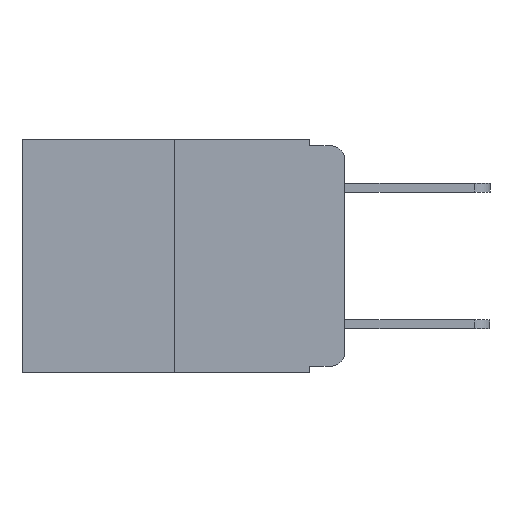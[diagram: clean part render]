
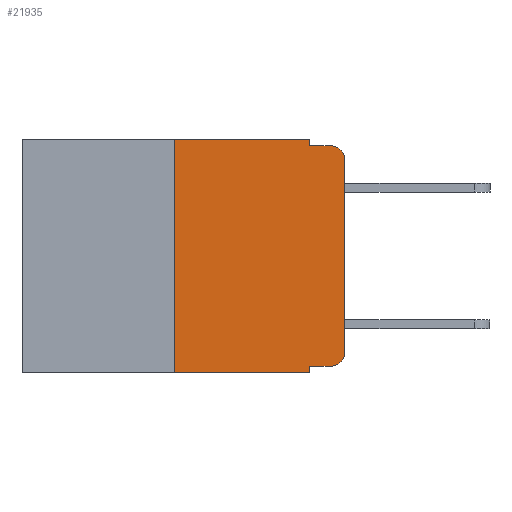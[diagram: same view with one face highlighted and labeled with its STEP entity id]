
A CAD part, left-side view. The second image highlights one B-rep face of the part: STEP entity #21935.
In plain terms, the highlighted planar face has unit normal (-1, 0, 0).
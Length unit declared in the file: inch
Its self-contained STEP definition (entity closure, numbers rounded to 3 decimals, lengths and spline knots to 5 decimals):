
#330 = ORIENTED_EDGE ( 'NONE', *, *, #23848, .F. ) ;
#462 = ORIENTED_EDGE ( 'NONE', *, *, #19338, .F. ) ;
#585 = CARTESIAN_POINT ( 'NONE',  ( 0., 0.051, -0.333 ) ) ;
#984 = ORIENTED_EDGE ( 'NONE', *, *, #8933, .F. ) ;
#1014 = AXIS2_PLACEMENT_3D ( 'NONE', #10440, #23750, #12468 ) ;
#1226 = ORIENTED_EDGE ( 'NONE', *, *, #25262, .T. ) ;
#1293 = ORIENTED_EDGE ( 'NONE', *, *, #23496, .F. ) ;
#1392 = VERTEX_POINT ( 'NONE', #13499 ) ;
#1711 = CARTESIAN_POINT ( 'NONE',  ( 0., 0.25, 0. ) ) ;
#1817 = ORIENTED_EDGE ( 'NONE', *, *, #15068, .F. ) ;
#2026 = DIRECTION ( 'NONE',  ( 0., -1., 0. ) ) ;
#2485 = EDGE_CURVE ( 'NONE', #4805, #18798, #21576, .T. ) ;
#2813 = CARTESIAN_POINT ( 'NONE',  ( 0., 0.051, -0.333 ) ) ;
#2828 = VERTEX_POINT ( 'NONE', #23928 ) ;
#3461 = DIRECTION ( 'NONE',  ( 0., 0., 1. ) ) ;
#3633 = ORIENTED_EDGE ( 'NONE', *, *, #18887, .T. ) ;
#3906 = CARTESIAN_POINT ( 'NONE',  ( 0., 0.051, -0.343 ) ) ;
#4302 = CARTESIAN_POINT ( 'NONE',  ( 0., 0.051, -0.01 ) ) ;
#4327 = LINE ( 'NONE', #13667, #20032 ) ;
#4404 = DIRECTION ( 'NONE',  ( 0., -1., 0. ) ) ;
#4767 = CARTESIAN_POINT ( 'NONE',  ( 0., 0.02, -0.333 ) ) ;
#4805 = VERTEX_POINT ( 'NONE', #2813 ) ;
#5631 = ORIENTED_EDGE ( 'NONE', *, *, #2485, .T. ) ;
#5801 = ORIENTED_EDGE ( 'NONE', *, *, #12604, .T. ) ;
#5936 = DIRECTION ( 'NONE',  ( 0., 0., 1. ) ) ;
#6118 = ORIENTED_EDGE ( 'NONE', *, *, #23809, .T. ) ;
#6268 = VECTOR ( 'NONE', #3461, 39.37008 ) ;
#8522 = CARTESIAN_POINT ( 'NONE',  ( 0., 0.02, -0.01 ) ) ;
#8933 = EDGE_CURVE ( 'NONE', #10217, #2828, #17634, .T. ) ;
#9386 = LINE ( 'NONE', #12485, #23977 ) ;
#9633 = LINE ( 'NONE', #18454, #23635 ) ;
#10127 = VERTEX_POINT ( 'NONE', #10165 ) ;
#10142 = DIRECTION ( 'NONE',  ( -1., 0., 0. ) ) ;
#10165 = CARTESIAN_POINT ( 'NONE',  ( 0., 0., -0.313 ) ) ;
#10217 = VERTEX_POINT ( 'NONE', #21862 ) ;
#10440 = CARTESIAN_POINT ( 'NONE',  ( 0., 0.473, 0. ) ) ;
#10537 = DIRECTION ( 'NONE',  ( 0., 0., -1. ) ) ;
#11030 = CIRCLE ( 'NONE', #16475, 0.02 ) ;
#11188 = DIRECTION ( 'NONE',  ( -1., 0., 0. ) ) ;
#11749 = FACE_OUTER_BOUND ( 'NONE', #16472, .T. ) ;
#12265 = VECTOR ( 'NONE', #10537, 39.37008 ) ;
#12468 = DIRECTION ( 'NONE',  ( 0., 0., -1. ) ) ;
#12481 = VECTOR ( 'NONE', #5936, 39.37008 ) ;
#12485 = CARTESIAN_POINT ( 'NONE',  ( 0., 0.473, -0.343 ) ) ;
#12543 = VERTEX_POINT ( 'NONE', #23163 ) ;
#12604 = EDGE_CURVE ( 'NONE', #18798, #10127, #11030, .T. ) ;
#13340 = VECTOR ( 'NONE', #2026, 39.37008 ) ;
#13499 = CARTESIAN_POINT ( 'NONE',  ( 0., 0.051, 0. ) ) ;
#13667 = CARTESIAN_POINT ( 'NONE',  ( 0., 0.473, 0. ) ) ;
#14614 = DIRECTION ( 'NONE',  ( 0., 0., -1. ) ) ;
#15068 = EDGE_CURVE ( 'NONE', #17751, #16183, #18084, .T. ) ;
#15530 = CARTESIAN_POINT ( 'NONE',  ( 0., 0., 0. ) ) ;
#15623 = DIRECTION ( 'NONE',  ( 0., -1., 0. ) ) ;
#16183 = VERTEX_POINT ( 'NONE', #8522 ) ;
#16472 = EDGE_LOOP ( 'NONE', ( #6118, #3633, #1817, #462, #330, #984, #1226, #1293, #5631, #5801 ) ) ;
#16475 = AXIS2_PLACEMENT_3D ( 'NONE', #21605, #10142, #23472 ) ;
#17267 = DIRECTION ( 'NONE',  ( 0., -1., 0. ) ) ;
#17341 = CARTESIAN_POINT ( 'NONE',  ( 0., 0.051, -0.01 ) ) ;
#17495 = VECTOR ( 'NONE', #17267, 39.37008 ) ;
#17634 = LINE ( 'NONE', #1711, #12481 ) ;
#17751 = VERTEX_POINT ( 'NONE', #4302 ) ;
#18084 = LINE ( 'NONE', #17341, #17495 ) ;
#18454 = CARTESIAN_POINT ( 'NONE',  ( 0., 0.051, 0. ) ) ;
#18595 = LINE ( 'NONE', #20118, #12265 ) ;
#18798 = VERTEX_POINT ( 'NONE', #4767 ) ;
#18887 = EDGE_CURVE ( 'NONE', #12543, #16183, #21073, .T. ) ;
#19338 = EDGE_CURVE ( 'NONE', #1392, #17751, #9633, .T. ) ;
#20032 = VECTOR ( 'NONE', #15623, 39.37008 ) ;
#20118 = CARTESIAN_POINT ( 'NONE',  ( 0., 0.051, 0. ) ) ;
#20217 = VERTEX_POINT ( 'NONE', #3906 ) ;
#21073 = CIRCLE ( 'NONE', #24005, 0.02 ) ;
#21576 = LINE ( 'NONE', #585, #13340 ) ;
#21605 = CARTESIAN_POINT ( 'NONE',  ( 0., 0.02, -0.313 ) ) ;
#21862 = CARTESIAN_POINT ( 'NONE',  ( 0., 0.25, -0.343 ) ) ;
#21877 = PLANE ( 'NONE',  #1014 ) ;
#21935 = ADVANCED_FACE ( 'NONE', ( #11749 ), #21877, .F. ) ;
#22555 = CARTESIAN_POINT ( 'NONE',  ( 0., 0.02, -0.03 ) ) ;
#23163 = CARTESIAN_POINT ( 'NONE',  ( 0., 0., -0.03 ) ) ;
#23472 = DIRECTION ( 'NONE',  ( 0., 0., -1. ) ) ;
#23496 = EDGE_CURVE ( 'NONE', #4805, #20217, #18595, .T. ) ;
#23635 = VECTOR ( 'NONE', #14614, 39.37008 ) ;
#23750 = DIRECTION ( 'NONE',  ( 1., 0., 0. ) ) ;
#23809 = EDGE_CURVE ( 'NONE', #10127, #12543, #24921, .T. ) ;
#23848 = EDGE_CURVE ( 'NONE', #2828, #1392, #4327, .T. ) ;
#23928 = CARTESIAN_POINT ( 'NONE',  ( 0., 0.25, 0. ) ) ;
#23977 = VECTOR ( 'NONE', #4404, 39.37008 ) ;
#24005 = AXIS2_PLACEMENT_3D ( 'NONE', #22555, #11188, #24404 ) ;
#24404 = DIRECTION ( 'NONE',  ( 0., 0., -1. ) ) ;
#24921 = LINE ( 'NONE', #15530, #6268 ) ;
#25262 = EDGE_CURVE ( 'NONE', #10217, #20217, #9386, .T. ) ;
